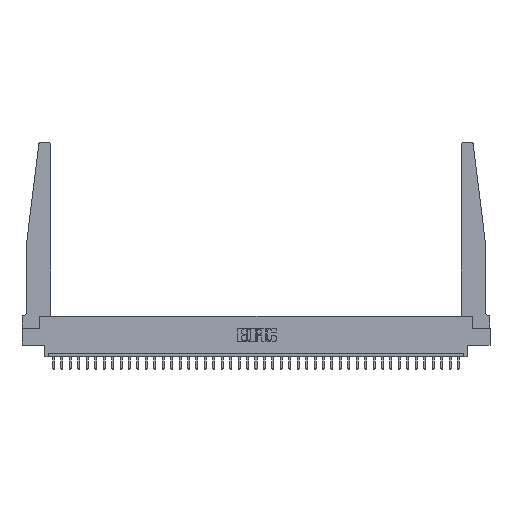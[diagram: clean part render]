
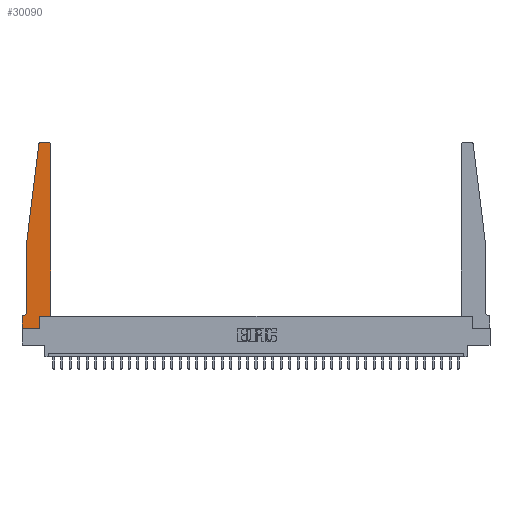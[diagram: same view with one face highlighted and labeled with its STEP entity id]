
A CAD part, top view. The second image highlights one B-rep face of the part: STEP entity #30090.
In plain terms, the highlighted planar face has unit normal (0, 0, 1).
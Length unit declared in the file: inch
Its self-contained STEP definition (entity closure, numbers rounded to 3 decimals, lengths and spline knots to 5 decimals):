
#15 = EDGE_CURVE ( 'NONE', #22167, #1829, #12402, .T. ) ;
#446 = VERTEX_POINT ( 'NONE', #9481 ) ;
#1318 = VECTOR ( 'NONE', #27962, 39.37008 ) ;
#1505 = VERTEX_POINT ( 'NONE', #11382 ) ;
#1763 = DIRECTION ( 'NONE',  ( -1., 0., 0. ) ) ;
#1829 = VERTEX_POINT ( 'NONE', #24209 ) ;
#1962 = ORIENTED_EDGE ( 'NONE', *, *, #6894, .T. ) ;
#2163 = DIRECTION ( 'NONE',  ( 0., 1., 0. ) ) ;
#2284 = ORIENTED_EDGE ( 'NONE', *, *, #15, .T. ) ;
#2504 = CARTESIAN_POINT ( 'NONE',  ( 0.25, 2.75, 0.37 ) ) ;
#2774 = AXIS2_PLACEMENT_3D ( 'NONE', #4576, #23254, #18199 ) ;
#3347 = ORIENTED_EDGE ( 'NONE', *, *, #12189, .T. ) ;
#3834 = DIRECTION ( 'NONE',  ( 0., -1., 0. ) ) ;
#4466 = VECTOR ( 'NONE', #5809, 39.37008 ) ;
#4576 = CARTESIAN_POINT ( 'NONE',  ( 0.015, 0.2375, 0.37 ) ) ;
#4625 = LINE ( 'NONE', #28953, #10878 ) ;
#5413 = VERTEX_POINT ( 'NONE', #31680 ) ;
#5809 = DIRECTION ( 'NONE',  ( 1., 0., 0. ) ) ;
#6081 = ORIENTED_EDGE ( 'NONE', *, *, #8613, .T. ) ;
#6122 = CARTESIAN_POINT ( 'NONE',  ( 0.2605, 0.18, 0.37 ) ) ;
#6580 = EDGE_LOOP ( 'NONE', ( #3347, #14080, #9194, #12255, #26954, #21847, #15538, #13146, #11275, #2284, #1962, #6081 ) ) ;
#6894 = EDGE_CURVE ( 'NONE', #1829, #5413, #31405, .T. ) ;
#6952 = DIRECTION ( 'NONE',  ( 1., 0., 0. ) ) ;
#7540 = LINE ( 'NONE', #25183, #10471 ) ;
#7579 = CARTESIAN_POINT ( 'NONE',  ( 0.395, 2.72, 0.37 ) ) ;
#8450 = VERTEX_POINT ( 'NONE', #30376 ) ;
#8613 = EDGE_CURVE ( 'NONE', #5413, #23251, #27151, .T. ) ;
#9194 = ORIENTED_EDGE ( 'NONE', *, *, #10011, .T. ) ;
#9461 = FACE_OUTER_BOUND ( 'NONE', #6580, .T. ) ;
#9481 = CARTESIAN_POINT ( 'NONE',  ( 0.065, 1.25, 0.37 ) ) ;
#10011 = EDGE_CURVE ( 'NONE', #16046, #446, #18786, .T. ) ;
#10471 = VECTOR ( 'NONE', #3834, 39.37008 ) ;
#10809 = CARTESIAN_POINT ( 'NONE',  ( 0., 0., 0.37 ) ) ;
#10878 = VECTOR ( 'NONE', #2163, 39.37008 ) ;
#11275 = ORIENTED_EDGE ( 'NONE', *, *, #20758, .T. ) ;
#11382 = CARTESIAN_POINT ( 'NONE',  ( 0.27653, 2.75, 0.37 ) ) ;
#12018 = DIRECTION ( 'NONE',  ( 0., 1., 0. ) ) ;
#12189 = EDGE_CURVE ( 'NONE', #23251, #1505, #34128, .T. ) ;
#12255 = ORIENTED_EDGE ( 'NONE', *, *, #24489, .T. ) ;
#12402 = LINE ( 'NONE', #21805, #4466 ) ;
#12915 = DIRECTION ( 'NONE',  ( 0., 0., 1. ) ) ;
#13146 = ORIENTED_EDGE ( 'NONE', *, *, #20107, .T. ) ;
#13816 = CARTESIAN_POINT ( 'NONE',  ( 0.065, 0.2375, 0.37 ) ) ;
#13857 = VECTOR ( 'NONE', #12018, 39.37008 ) ;
#14080 = ORIENTED_EDGE ( 'NONE', *, *, #31554, .T. ) ;
#15297 = CARTESIAN_POINT ( 'NONE',  ( 0.395, 2.75, 0.37 ) ) ;
#15538 = ORIENTED_EDGE ( 'NONE', *, *, #20364, .T. ) ;
#15671 = PLANE ( 'NONE',  #31156 ) ;
#15910 = DIRECTION ( 'NONE',  ( -1., 0., 0. ) ) ;
#16046 = VERTEX_POINT ( 'NONE', #31126 ) ;
#16805 = VECTOR ( 'NONE', #25851, 39.37008 ) ;
#17055 = VECTOR ( 'NONE', #15910, 39.37008 ) ;
#17209 = CIRCLE ( 'NONE', #2774, 0.05 ) ;
#17553 = CARTESIAN_POINT ( 'NONE',  ( 0.2605, 0., 0.37 ) ) ;
#18199 = DIRECTION ( 'NONE',  ( -1., 0., 0. ) ) ;
#18289 = CARTESIAN_POINT ( 'NONE',  ( 0., 0., 0.37 ) ) ;
#18786 = LINE ( 'NONE', #33203, #1318 ) ;
#18985 = VERTEX_POINT ( 'NONE', #23715 ) ;
#19697 = EDGE_CURVE ( 'NONE', #25551, #18985, #17209, .T. ) ;
#20107 = EDGE_CURVE ( 'NONE', #27543, #29950, #20955, .T. ) ;
#20364 = EDGE_CURVE ( 'NONE', #8450, #27543, #7540, .T. ) ;
#20758 = EDGE_CURVE ( 'NONE', #29950, #22167, #4625, .T. ) ;
#20955 = LINE ( 'NONE', #10809, #22215 ) ;
#21779 = DIRECTION ( 'NONE',  ( 1., 0., 0. ) ) ;
#21805 = CARTESIAN_POINT ( 'NONE',  ( 0.425, 0.18, 0.37 ) ) ;
#21847 = ORIENTED_EDGE ( 'NONE', *, *, #34192, .T. ) ;
#22167 = VERTEX_POINT ( 'NONE', #6122 ) ;
#22215 = VECTOR ( 'NONE', #21779, 39.37008 ) ;
#23145 = DIRECTION ( 'NONE',  ( 1., 0., 0. ) ) ;
#23251 = VERTEX_POINT ( 'NONE', #15297 ) ;
#23254 = DIRECTION ( 'NONE',  ( 0., 0., -1. ) ) ;
#23380 = DIRECTION ( 'NONE',  ( 0., 0., 1. ) ) ;
#23695 = AXIS2_PLACEMENT_3D ( 'NONE', #7579, #23380, #23145 ) ;
#23715 = CARTESIAN_POINT ( 'NONE',  ( 0.015, 0.1875, 0.37 ) ) ;
#24041 = CIRCLE ( 'NONE', #33651, 0.03 ) ;
#24209 = CARTESIAN_POINT ( 'NONE',  ( 0.425, 0.18, 0.37 ) ) ;
#24489 = EDGE_CURVE ( 'NONE', #446, #25551, #27679, .T. ) ;
#24541 = LINE ( 'NONE', #25429, #30769 ) ;
#25183 = CARTESIAN_POINT ( 'NONE',  ( 0., 0., 0.37 ) ) ;
#25429 = CARTESIAN_POINT ( 'NONE',  ( 0.065, 0.1875, 0.37 ) ) ;
#25551 = VERTEX_POINT ( 'NONE', #13816 ) ;
#25851 = DIRECTION ( 'NONE',  ( 0., -1., 0. ) ) ;
#26198 = DIRECTION ( 'NONE',  ( 0., 0., 1. ) ) ;
#26954 = ORIENTED_EDGE ( 'NONE', *, *, #19697, .T. ) ;
#27151 = CIRCLE ( 'NONE', #23695, 0.03 ) ;
#27543 = VERTEX_POINT ( 'NONE', #18289 ) ;
#27679 = LINE ( 'NONE', #33880, #16805 ) ;
#27962 = DIRECTION ( 'NONE',  ( -0.122, -0.992, 0. ) ) ;
#28000 = CARTESIAN_POINT ( 'NONE',  ( 0.425, 0.18, 0.37 ) ) ;
#28877 = CARTESIAN_POINT ( 'NONE',  ( 0.27653, 2.72, 0.37 ) ) ;
#28953 = CARTESIAN_POINT ( 'NONE',  ( 0.2605, 0.18, 0.37 ) ) ;
#29950 = VERTEX_POINT ( 'NONE', #17553 ) ;
#30090 = ADVANCED_FACE ( 'NONE', ( #9461 ), #15671, .T. ) ;
#30376 = CARTESIAN_POINT ( 'NONE',  ( 0., 0.1875, 0.37 ) ) ;
#30769 = VECTOR ( 'NONE', #1763, 39.37008 ) ;
#31126 = CARTESIAN_POINT ( 'NONE',  ( 0.24675, 2.72367, 0.37 ) ) ;
#31156 = AXIS2_PLACEMENT_3D ( 'NONE', #34324, #26198, #31534 ) ;
#31405 = LINE ( 'NONE', #28000, #13857 ) ;
#31534 = DIRECTION ( 'NONE',  ( 1., 0., 0. ) ) ;
#31554 = EDGE_CURVE ( 'NONE', #1505, #16046, #24041, .T. ) ;
#31680 = CARTESIAN_POINT ( 'NONE',  ( 0.425, 2.72, 0.37 ) ) ;
#33203 = CARTESIAN_POINT ( 'NONE',  ( 0.065, 1.25, 0.37 ) ) ;
#33651 = AXIS2_PLACEMENT_3D ( 'NONE', #28877, #12915, #6952 ) ;
#33880 = CARTESIAN_POINT ( 'NONE',  ( 0.065, 1.25, 0.37 ) ) ;
#34128 = LINE ( 'NONE', #2504, #17055 ) ;
#34192 = EDGE_CURVE ( 'NONE', #18985, #8450, #24541, .T. ) ;
#34324 = CARTESIAN_POINT ( 'NONE',  ( 0., 0.1875, 0.37 ) ) ;
